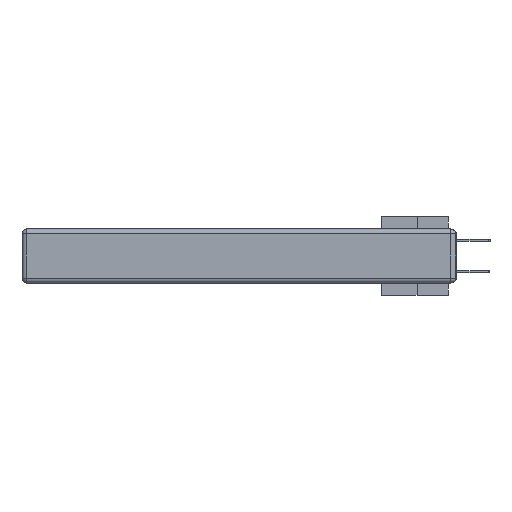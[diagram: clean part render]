
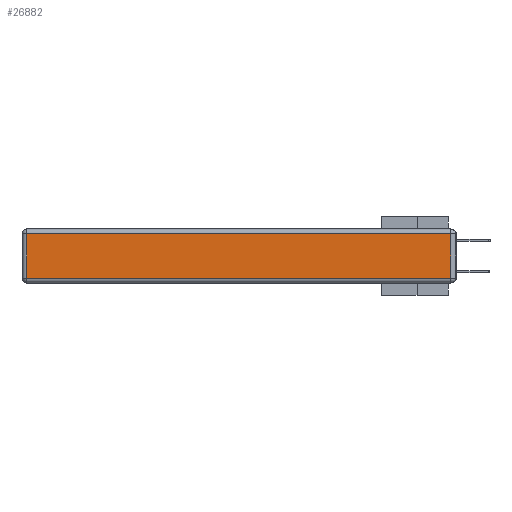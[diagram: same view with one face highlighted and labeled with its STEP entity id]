
A CAD part, left-side view. The second image highlights one B-rep face of the part: STEP entity #26882.
In plain terms, the highlighted planar face has unit normal (-1, 0, 0).
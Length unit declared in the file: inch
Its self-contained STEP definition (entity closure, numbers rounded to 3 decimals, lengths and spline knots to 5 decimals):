
#841 = VERTEX_POINT ( 'NONE', #19563 ) ;
#1729 = EDGE_CURVE ( 'NONE', #12136, #17295, #15184, .T. ) ;
#4895 = CARTESIAN_POINT ( 'NONE',  ( 0., 0., -0.343 ) ) ;
#5421 = EDGE_LOOP ( 'NONE', ( #7542, #8038, #16908, #17921 ) ) ;
#5494 = AXIS2_PLACEMENT_3D ( 'NONE', #4895, #9850, #18581 ) ;
#5572 = VECTOR ( 'NONE', #11747, 39.37008 ) ;
#5919 = CARTESIAN_POINT ( 'NONE',  ( 0., 0.03, -0.03 ) ) ;
#7298 = CARTESIAN_POINT ( 'NONE',  ( 0., 2.75, -0.03 ) ) ;
#7542 = ORIENTED_EDGE ( 'NONE', *, *, #16293, .T. ) ;
#7558 = PLANE ( 'NONE',  #5494 ) ;
#7793 = DIRECTION ( 'NONE',  ( 0., 0., -1. ) ) ;
#8038 = ORIENTED_EDGE ( 'NONE', *, *, #1729, .T. ) ;
#8192 = CARTESIAN_POINT ( 'NONE',  ( 0., 0.03, -0.313 ) ) ;
#9333 = VERTEX_POINT ( 'NONE', #22561 ) ;
#9850 = DIRECTION ( 'NONE',  ( -1., 0., 0. ) ) ;
#9863 = LINE ( 'NONE', #12434, #14832 ) ;
#10589 = VECTOR ( 'NONE', #14624, 39.37008 ) ;
#11578 = LINE ( 'NONE', #7298, #5572 ) ;
#11747 = DIRECTION ( 'NONE',  ( 0., 1., 0. ) ) ;
#12136 = VERTEX_POINT ( 'NONE', #8192 ) ;
#12434 = CARTESIAN_POINT ( 'NONE',  ( 0., 0., -0.313 ) ) ;
#14624 = DIRECTION ( 'NONE',  ( 0., 0., 1. ) ) ;
#14656 = VECTOR ( 'NONE', #7793, 39.37008 ) ;
#14832 = VECTOR ( 'NONE', #21491, 39.37008 ) ;
#15184 = LINE ( 'NONE', #28219, #10589 ) ;
#16293 = EDGE_CURVE ( 'NONE', #9333, #12136, #9863, .T. ) ;
#16908 = ORIENTED_EDGE ( 'NONE', *, *, #17027, .T. ) ;
#17027 = EDGE_CURVE ( 'NONE', #17295, #841, #11578, .T. ) ;
#17295 = VERTEX_POINT ( 'NONE', #5919 ) ;
#17921 = ORIENTED_EDGE ( 'NONE', *, *, #26407, .T. ) ;
#18581 = DIRECTION ( 'NONE',  ( 0., 0., 1. ) ) ;
#19306 = LINE ( 'NONE', #21205, #14656 ) ;
#19563 = CARTESIAN_POINT ( 'NONE',  ( 0., 2.72, -0.03 ) ) ;
#21205 = CARTESIAN_POINT ( 'NONE',  ( 0., 2.72, -0.343 ) ) ;
#21491 = DIRECTION ( 'NONE',  ( 0., -1., 0. ) ) ;
#22561 = CARTESIAN_POINT ( 'NONE',  ( 0., 2.72, -0.313 ) ) ;
#26377 = FACE_OUTER_BOUND ( 'NONE', #5421, .T. ) ;
#26407 = EDGE_CURVE ( 'NONE', #841, #9333, #19306, .T. ) ;
#26882 = ADVANCED_FACE ( 'NONE', ( #26377 ), #7558, .T. ) ;
#28219 = CARTESIAN_POINT ( 'NONE',  ( 0., 0.03, -0.343 ) ) ;
